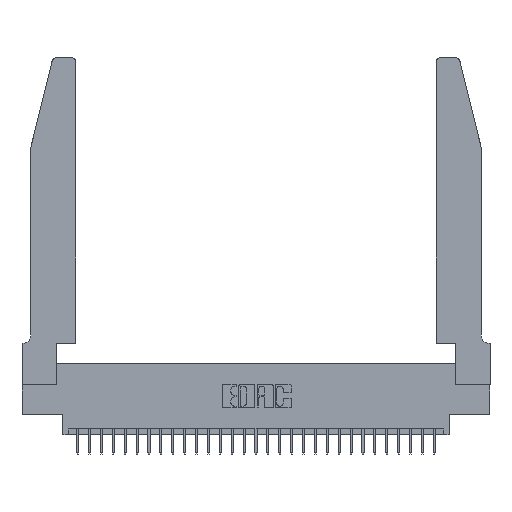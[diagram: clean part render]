
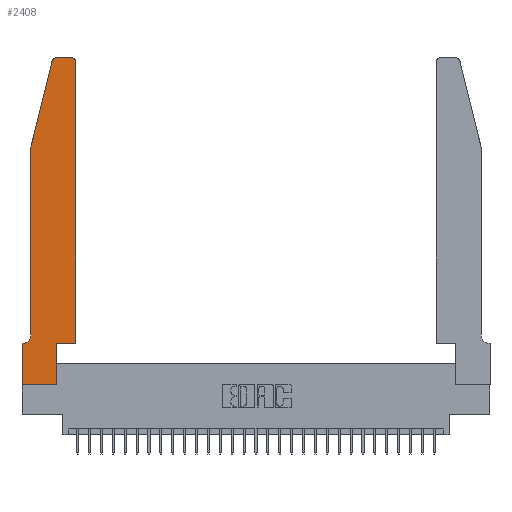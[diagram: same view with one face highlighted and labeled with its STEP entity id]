
A CAD part, top view. The second image highlights one B-rep face of the part: STEP entity #2408.
In plain terms, the highlighted planar face has unit normal (0, 0, 1).
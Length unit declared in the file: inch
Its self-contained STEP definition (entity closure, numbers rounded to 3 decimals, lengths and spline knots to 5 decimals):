
#103 = LINE ( 'NONE', #13484, #13144 ) ;
#220 = ORIENTED_EDGE ( 'NONE', *, *, #11457, .T. ) ;
#276 = CARTESIAN_POINT ( 'NONE',  ( 0., 0., 0.37 ) ) ;
#377 = DIRECTION ( 'NONE',  ( -1., 0., 0. ) ) ;
#535 = VERTEX_POINT ( 'NONE', #30202 ) ;
#949 = DIRECTION ( 'NONE',  ( 0., 1., 0. ) ) ;
#1103 = VECTOR ( 'NONE', #17310, 39.37008 ) ;
#1367 = ORIENTED_EDGE ( 'NONE', *, *, #13919, .T. ) ;
#1388 = CIRCLE ( 'NONE', #14603, 0.03 ) ;
#1675 = VERTEX_POINT ( 'NONE', #4105 ) ;
#1737 = VERTEX_POINT ( 'NONE', #13941 ) ;
#2217 = ORIENTED_EDGE ( 'NONE', *, *, #9059, .T. ) ;
#2408 = ADVANCED_FACE ( 'NONE', ( #14270 ), #20687, .T. ) ;
#2534 = EDGE_CURVE ( 'NONE', #17540, #22612, #16884, .T. ) ;
#2642 = ORIENTED_EDGE ( 'NONE', *, *, #17492, .T. ) ;
#2824 = CARTESIAN_POINT ( 'NONE',  ( 0.4505, 2.72, 0.37 ) ) ;
#4105 = CARTESIAN_POINT ( 'NONE',  ( 0.2865, 0.35, 0.37 ) ) ;
#4175 = CARTESIAN_POINT ( 'NONE',  ( 0., 0.35, 0.37 ) ) ;
#4259 = AXIS2_PLACEMENT_3D ( 'NONE', #4616, #21293, #7045 ) ;
#4572 = ORIENTED_EDGE ( 'NONE', *, *, #20892, .T. ) ;
#4616 = CARTESIAN_POINT ( 'NONE',  ( 0.4205, 2.72, 0.37 ) ) ;
#5481 = VECTOR ( 'NONE', #27472, 39.37008 ) ;
#5564 = CARTESIAN_POINT ( 'NONE',  ( 0.0755, 2., 0.37 ) ) ;
#6627 = DIRECTION ( 'NONE',  ( 1., 0., 0. ) ) ;
#7018 = VERTEX_POINT ( 'NONE', #14396 ) ;
#7045 = DIRECTION ( 'NONE',  ( 1., 0., 0. ) ) ;
#7064 = CARTESIAN_POINT ( 'NONE',  ( 0.4205, 2.75, 0.37 ) ) ;
#7560 = ORIENTED_EDGE ( 'NONE', *, *, #26484, .T. ) ;
#8175 = EDGE_CURVE ( 'NONE', #7018, #17540, #21415, .T. ) ;
#8436 = VERTEX_POINT ( 'NONE', #5564 ) ;
#8610 = VECTOR ( 'NONE', #20862, 39.37008 ) ;
#9059 = EDGE_CURVE ( 'NONE', #29983, #535, #22771, .T. ) ;
#9268 = DIRECTION ( 'NONE',  ( 0., 1., 0. ) ) ;
#9503 = ORIENTED_EDGE ( 'NONE', *, *, #21292, .T. ) ;
#9570 = VECTOR ( 'NONE', #9268, 39.37008 ) ;
#9840 = CARTESIAN_POINT ( 'NONE',  ( 0.0755, 0.42, 0.37 ) ) ;
#9853 = DIRECTION ( 'NONE',  ( 1., 0., 0. ) ) ;
#9926 = VERTEX_POINT ( 'NONE', #15549 ) ;
#10450 = CARTESIAN_POINT ( 'NONE',  ( 0.284, 2.72, 0.37 ) ) ;
#10962 = CARTESIAN_POINT ( 'NONE',  ( 0.2865, 0., 0.37 ) ) ;
#11374 = CARTESIAN_POINT ( 'NONE',  ( 0., 0., 0.37 ) ) ;
#11457 = EDGE_CURVE ( 'NONE', #9926, #8436, #12681, .T. ) ;
#12314 = EDGE_CURVE ( 'NONE', #1737, #17174, #19625, .T. ) ;
#12681 = LINE ( 'NONE', #22874, #5481 ) ;
#12880 = DIRECTION ( 'NONE',  ( 1., 0., 0. ) ) ;
#13144 = VECTOR ( 'NONE', #15877, 39.37008 ) ;
#13221 = CARTESIAN_POINT ( 'NONE',  ( 0., 0.35, 0.37 ) ) ;
#13484 = CARTESIAN_POINT ( 'NONE',  ( 0.2605, 2.75, 0.37 ) ) ;
#13919 = EDGE_CURVE ( 'NONE', #13959, #9926, #1388, .T. ) ;
#13941 = CARTESIAN_POINT ( 'NONE',  ( 0., 0., 0.37 ) ) ;
#13959 = VERTEX_POINT ( 'NONE', #22296 ) ;
#14270 = FACE_OUTER_BOUND ( 'NONE', #14847, .T. ) ;
#14396 = CARTESIAN_POINT ( 'NONE',  ( 0.4505, 0.35, 0.37 ) ) ;
#14603 = AXIS2_PLACEMENT_3D ( 'NONE', #10450, #26776, #12880 ) ;
#14847 = EDGE_LOOP ( 'NONE', ( #7560, #1367, #220, #21712, #2217, #9503, #4572, #26360, #2642, #28558, #18466, #25277 ) ) ;
#15025 = DIRECTION ( 'NONE',  ( 0., 0., -1. ) ) ;
#15074 = EDGE_CURVE ( 'NONE', #8436, #29983, #15417, .T. ) ;
#15417 = LINE ( 'NONE', #21540, #26967 ) ;
#15549 = CARTESIAN_POINT ( 'NONE',  ( 0.25487, 2.72718, 0.37 ) ) ;
#15877 = DIRECTION ( 'NONE',  ( -1., 0., 0. ) ) ;
#16343 = EDGE_CURVE ( 'NONE', #1675, #7018, #17251, .T. ) ;
#16884 = CIRCLE ( 'NONE', #4259, 0.03 ) ;
#17076 = LINE ( 'NONE', #29390, #28597 ) ;
#17174 = VERTEX_POINT ( 'NONE', #10962 ) ;
#17251 = LINE ( 'NONE', #21629, #23372 ) ;
#17310 = DIRECTION ( 'NONE',  ( 1., 0., 0. ) ) ;
#17492 = EDGE_CURVE ( 'NONE', #17174, #1675, #17076, .T. ) ;
#17540 = VERTEX_POINT ( 'NONE', #2824 ) ;
#18368 = LINE ( 'NONE', #11374, #24500 ) ;
#18466 = ORIENTED_EDGE ( 'NONE', *, *, #8175, .T. ) ;
#19566 = VERTEX_POINT ( 'NONE', #13221 ) ;
#19625 = LINE ( 'NONE', #276, #1103 ) ;
#20529 = LINE ( 'NONE', #20769, #8610 ) ;
#20687 = PLANE ( 'NONE',  #30101 ) ;
#20769 = CARTESIAN_POINT ( 'NONE',  ( 0.0755, 0.35, 0.37 ) ) ;
#20862 = DIRECTION ( 'NONE',  ( -1., 0., 0. ) ) ;
#20887 = DIRECTION ( 'NONE',  ( 0., 0., 1. ) ) ;
#20892 = EDGE_CURVE ( 'NONE', #19566, #1737, #18368, .T. ) ;
#21292 = EDGE_CURVE ( 'NONE', #535, #19566, #20529, .T. ) ;
#21293 = DIRECTION ( 'NONE',  ( 0., 0., 1. ) ) ;
#21415 = LINE ( 'NONE', #27893, #9570 ) ;
#21540 = CARTESIAN_POINT ( 'NONE',  ( 0.0755, 2., 0.37 ) ) ;
#21629 = CARTESIAN_POINT ( 'NONE',  ( 0.4505, 0.35, 0.37 ) ) ;
#21712 = ORIENTED_EDGE ( 'NONE', *, *, #15074, .T. ) ;
#22296 = CARTESIAN_POINT ( 'NONE',  ( 0.284, 2.75, 0.37 ) ) ;
#22612 = VERTEX_POINT ( 'NONE', #7064 ) ;
#22771 = CIRCLE ( 'NONE', #28884, 0.07 ) ;
#22874 = CARTESIAN_POINT ( 'NONE',  ( 0.0755, 2., 0.37 ) ) ;
#23372 = VECTOR ( 'NONE', #9853, 39.37008 ) ;
#24500 = VECTOR ( 'NONE', #27633, 39.37008 ) ;
#25277 = ORIENTED_EDGE ( 'NONE', *, *, #2534, .T. ) ;
#26113 = DIRECTION ( 'NONE',  ( 0., -1., 0. ) ) ;
#26360 = ORIENTED_EDGE ( 'NONE', *, *, #12314, .T. ) ;
#26484 = EDGE_CURVE ( 'NONE', #22612, #13959, #103, .T. ) ;
#26776 = DIRECTION ( 'NONE',  ( 0., 0., 1. ) ) ;
#26967 = VECTOR ( 'NONE', #26113, 39.37008 ) ;
#27472 = DIRECTION ( 'NONE',  ( -0.239, -0.971, 0. ) ) ;
#27633 = DIRECTION ( 'NONE',  ( 0., -1., 0. ) ) ;
#27893 = CARTESIAN_POINT ( 'NONE',  ( 0.4505, 0.35, 0.37 ) ) ;
#28558 = ORIENTED_EDGE ( 'NONE', *, *, #16343, .T. ) ;
#28597 = VECTOR ( 'NONE', #949, 39.37008 ) ;
#28875 = CARTESIAN_POINT ( 'NONE',  ( 0.0055, 0.42, 0.37 ) ) ;
#28884 = AXIS2_PLACEMENT_3D ( 'NONE', #28875, #15025, #377 ) ;
#29390 = CARTESIAN_POINT ( 'NONE',  ( 0.2865, 0.35, 0.37 ) ) ;
#29983 = VERTEX_POINT ( 'NONE', #9840 ) ;
#30101 = AXIS2_PLACEMENT_3D ( 'NONE', #4175, #20887, #6627 ) ;
#30202 = CARTESIAN_POINT ( 'NONE',  ( 0.0055, 0.35, 0.37 ) ) ;
